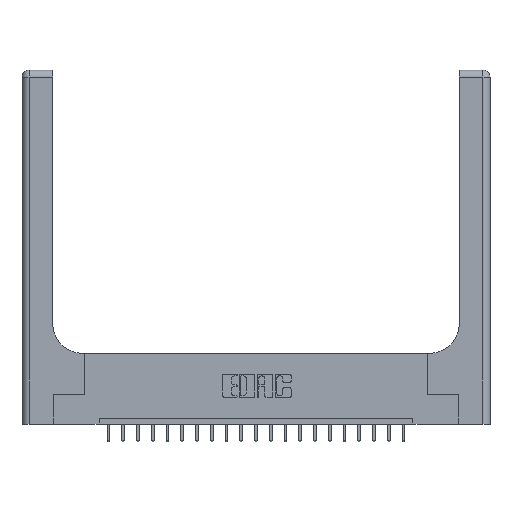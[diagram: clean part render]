
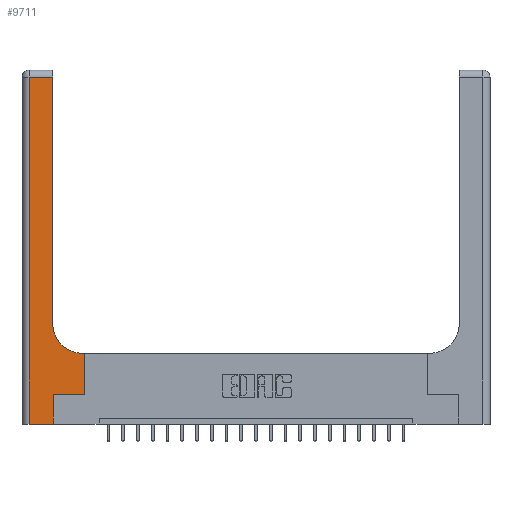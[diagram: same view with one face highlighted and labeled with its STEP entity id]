
A CAD part, top view. The second image highlights one B-rep face of the part: STEP entity #9711.
In plain terms, the highlighted planar face has unit normal (0, 0, 1).
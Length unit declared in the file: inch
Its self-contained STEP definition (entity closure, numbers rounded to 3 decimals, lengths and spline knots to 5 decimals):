
#25 = VECTOR ( 'NONE', #12476, 39.37008 ) ;
#73 = VERTEX_POINT ( 'NONE', #16270 ) ;
#623 = LINE ( 'NONE', #9095, #6211 ) ;
#897 = DIRECTION ( 'NONE',  ( 0., 0., -1. ) ) ;
#2105 = EDGE_CURVE ( 'NONE', #18962, #10917, #15524, .T. ) ;
#2309 = VERTEX_POINT ( 'NONE', #3101 ) ;
#2450 = CARTESIAN_POINT ( 'NONE',  ( 0.51, 0.85, 0.37 ) ) ;
#2491 = CARTESIAN_POINT ( 'NONE',  ( 0.528, 0.25, 0.37 ) ) ;
#3079 = ORIENTED_EDGE ( 'NONE', *, *, #6730, .T. ) ;
#3101 = CARTESIAN_POINT ( 'NONE',  ( 0.528, 0.25, 0.37 ) ) ;
#3340 = CARTESIAN_POINT ( 'NONE',  ( 0.265, 0., 0.37 ) ) ;
#3341 = ORIENTED_EDGE ( 'NONE', *, *, #2105, .T. ) ;
#4229 = ORIENTED_EDGE ( 'NONE', *, *, #10692, .T. ) ;
#4298 = VERTEX_POINT ( 'NONE', #12018 ) ;
#4699 = EDGE_CURVE ( 'NONE', #15254, #12609, #15759, .T. ) ;
#4961 = ORIENTED_EDGE ( 'NONE', *, *, #4699, .T. ) ;
#5241 = VECTOR ( 'NONE', #13688, 39.37008 ) ;
#5605 = EDGE_CURVE ( 'NONE', #18090, #2309, #17558, .T. ) ;
#5819 = CARTESIAN_POINT ( 'NONE',  ( 0.265, 0., 0.37 ) ) ;
#5843 = VECTOR ( 'NONE', #9532, 39.37008 ) ;
#6211 = VECTOR ( 'NONE', #11916, 39.37008 ) ;
#6258 = DIRECTION ( 'NONE',  ( -1., 0., 0. ) ) ;
#6667 = ORIENTED_EDGE ( 'NONE', *, *, #12856, .T. ) ;
#6730 = EDGE_CURVE ( 'NONE', #16707, #73, #623, .T. ) ;
#6807 = CARTESIAN_POINT ( 'NONE',  ( 0.26, 3., 0.37 ) ) ;
#7179 = CARTESIAN_POINT ( 'NONE',  ( 0.51, 0.6, 0.37 ) ) ;
#8292 = VECTOR ( 'NONE', #20083, 39.37008 ) ;
#9095 = CARTESIAN_POINT ( 'NONE',  ( 0., 2.94, 0.37 ) ) ;
#9416 = DIRECTION ( 'NONE',  ( 1., 0., 0. ) ) ;
#9532 = DIRECTION ( 'NONE',  ( 0., 1., 0. ) ) ;
#9711 = ADVANCED_FACE ( 'NONE', ( #14132 ), #19055, .F. ) ;
#10168 = CARTESIAN_POINT ( 'NONE',  ( 0.26, 0.85, 0.37 ) ) ;
#10359 = CARTESIAN_POINT ( 'NONE',  ( 0.06, 3., 0.37 ) ) ;
#10643 = EDGE_CURVE ( 'NONE', #4298, #18962, #18201, .T. ) ;
#10692 = EDGE_CURVE ( 'NONE', #12609, #18090, #16364, .T. ) ;
#10772 = CARTESIAN_POINT ( 'NONE',  ( 0., 0., 0.37 ) ) ;
#10917 = VERTEX_POINT ( 'NONE', #10168 ) ;
#11299 = ORIENTED_EDGE ( 'NONE', *, *, #10643, .T. ) ;
#11576 = CARTESIAN_POINT ( 'NONE',  ( 0.26, 0.6, 0.37 ) ) ;
#11691 = LINE ( 'NONE', #6807, #8292 ) ;
#11797 = ORIENTED_EDGE ( 'NONE', *, *, #5605, .T. ) ;
#11873 = LINE ( 'NONE', #10359, #17965 ) ;
#11916 = DIRECTION ( 'NONE',  ( -1., 0., 0. ) ) ;
#11997 = DIRECTION ( 'NONE',  ( 0., 0., -1. ) ) ;
#12018 = CARTESIAN_POINT ( 'NONE',  ( 0.528, 0.6, 0.37 ) ) ;
#12090 = VECTOR ( 'NONE', #9416, 39.37008 ) ;
#12476 = DIRECTION ( 'NONE',  ( 0., 1., 0. ) ) ;
#12609 = VERTEX_POINT ( 'NONE', #5819 ) ;
#12756 = EDGE_LOOP ( 'NONE', ( #13070, #3079, #6667, #4961, #4229, #11797, #13212, #11299, #3341 ) ) ;
#12856 = EDGE_CURVE ( 'NONE', #73, #15254, #11873, .T. ) ;
#13070 = ORIENTED_EDGE ( 'NONE', *, *, #14171, .T. ) ;
#13212 = ORIENTED_EDGE ( 'NONE', *, *, #16730, .T. ) ;
#13688 = DIRECTION ( 'NONE',  ( 1., 0., 0. ) ) ;
#14132 = FACE_OUTER_BOUND ( 'NONE', #12756, .T. ) ;
#14171 = EDGE_CURVE ( 'NONE', #10917, #16707, #11691, .T. ) ;
#14237 = CARTESIAN_POINT ( 'NONE',  ( 0., 3., 0.37 ) ) ;
#14410 = LINE ( 'NONE', #2491, #25 ) ;
#15254 = VERTEX_POINT ( 'NONE', #21211 ) ;
#15524 = CIRCLE ( 'NONE', #18656, 0.25 ) ;
#15759 = LINE ( 'NONE', #10772, #5241 ) ;
#15814 = CARTESIAN_POINT ( 'NONE',  ( 0.265, 0.25, 0.37 ) ) ;
#16270 = CARTESIAN_POINT ( 'NONE',  ( 0.06, 2.94, 0.37 ) ) ;
#16364 = LINE ( 'NONE', #3340, #5843 ) ;
#16698 = AXIS2_PLACEMENT_3D ( 'NONE', #14237, #897, #20906 ) ;
#16707 = VERTEX_POINT ( 'NONE', #19444 ) ;
#16730 = EDGE_CURVE ( 'NONE', #2309, #4298, #14410, .T. ) ;
#17558 = LINE ( 'NONE', #15814, #12090 ) ;
#17965 = VECTOR ( 'NONE', #18729, 39.37008 ) ;
#18090 = VERTEX_POINT ( 'NONE', #19367 ) ;
#18201 = LINE ( 'NONE', #11576, #19277 ) ;
#18656 = AXIS2_PLACEMENT_3D ( 'NONE', #2450, #11997, #20499 ) ;
#18729 = DIRECTION ( 'NONE',  ( 0., -1., 0. ) ) ;
#18962 = VERTEX_POINT ( 'NONE', #7179 ) ;
#19055 = PLANE ( 'NONE',  #16698 ) ;
#19277 = VECTOR ( 'NONE', #6258, 39.37008 ) ;
#19367 = CARTESIAN_POINT ( 'NONE',  ( 0.265, 0.25, 0.37 ) ) ;
#19444 = CARTESIAN_POINT ( 'NONE',  ( 0.26, 2.94, 0.37 ) ) ;
#20083 = DIRECTION ( 'NONE',  ( 0., 1., 0. ) ) ;
#20499 = DIRECTION ( 'NONE',  ( 1., 0., 0. ) ) ;
#20906 = DIRECTION ( 'NONE',  ( -1., 0., 0. ) ) ;
#21211 = CARTESIAN_POINT ( 'NONE',  ( 0.06, 0., 0.37 ) ) ;
